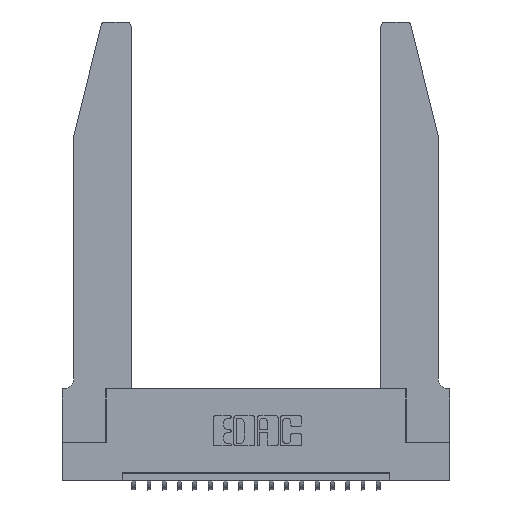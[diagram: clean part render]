
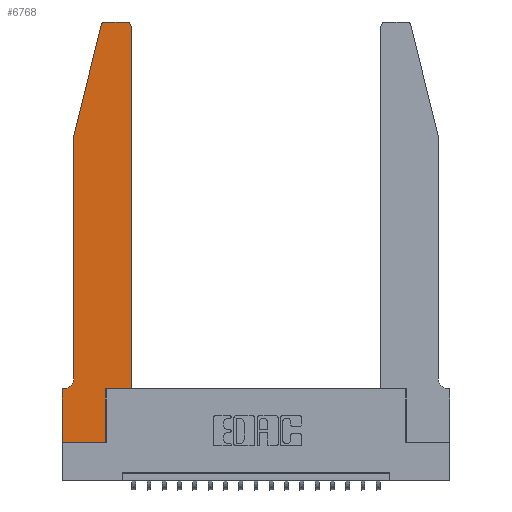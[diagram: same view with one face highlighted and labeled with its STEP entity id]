
A CAD part, top view. The second image highlights one B-rep face of the part: STEP entity #6768.
In plain terms, the highlighted planar face has unit normal (0, 0, 1).
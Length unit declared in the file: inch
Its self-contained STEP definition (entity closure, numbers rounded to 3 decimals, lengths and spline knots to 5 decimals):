
#66 = EDGE_CURVE ( 'NONE', #9543, #18279, #16035, .T. ) ;
#221 = VERTEX_POINT ( 'NONE', #3979 ) ;
#252 = DIRECTION ( 'NONE',  ( 0., -1., 0. ) ) ;
#942 = VERTEX_POINT ( 'NONE', #6035 ) ;
#1157 = CARTESIAN_POINT ( 'NONE',  ( 0.2865, 0., 0.37 ) ) ;
#1265 = EDGE_CURVE ( 'NONE', #18279, #14429, #11184, .T. ) ;
#2104 = ORIENTED_EDGE ( 'NONE', *, *, #1265, .T. ) ;
#2162 = LINE ( 'NONE', #9368, #5380 ) ;
#2373 = LINE ( 'NONE', #16168, #3080 ) ;
#2887 = CARTESIAN_POINT ( 'NONE',  ( 0., 0., 0.37 ) ) ;
#2983 = PLANE ( 'NONE',  #10038 ) ;
#3080 = VECTOR ( 'NONE', #16244, 39.37008 ) ;
#3248 = VERTEX_POINT ( 'NONE', #12413 ) ;
#3618 = CARTESIAN_POINT ( 'NONE',  ( 0.25487, 2.72718, 0.37 ) ) ;
#3940 = LINE ( 'NONE', #19467, #20176 ) ;
#3979 = CARTESIAN_POINT ( 'NONE',  ( 0., 0.35, 0.37 ) ) ;
#4299 = VECTOR ( 'NONE', #18456, 39.37008 ) ;
#4621 = EDGE_CURVE ( 'NONE', #221, #20211, #2162, .T. ) ;
#4654 = DIRECTION ( 'NONE',  ( 1., 0., 0. ) ) ;
#4764 = CARTESIAN_POINT ( 'NONE',  ( 0.0755, 0.42, 0.37 ) ) ;
#4888 = DIRECTION ( 'NONE',  ( -1., 0., 0. ) ) ;
#5045 = VECTOR ( 'NONE', #11213, 39.37008 ) ;
#5380 = VECTOR ( 'NONE', #20768, 39.37008 ) ;
#5398 = ORIENTED_EDGE ( 'NONE', *, *, #6050, .T. ) ;
#5723 = CARTESIAN_POINT ( 'NONE',  ( 0.0755, 2., 0.37 ) ) ;
#6035 = CARTESIAN_POINT ( 'NONE',  ( 0.4505, 0.35, 0.37 ) ) ;
#6050 = EDGE_CURVE ( 'NONE', #15713, #9543, #6128, .T. ) ;
#6083 = ORIENTED_EDGE ( 'NONE', *, *, #11339, .T. ) ;
#6128 = CIRCLE ( 'NONE', #12092, 0.03 ) ;
#6202 = DIRECTION ( 'NONE',  ( 0., 0., 1. ) ) ;
#6313 = CARTESIAN_POINT ( 'NONE',  ( 0.0755, 2., 0.37 ) ) ;
#6392 = ORIENTED_EDGE ( 'NONE', *, *, #66, .T. ) ;
#6768 = ADVANCED_FACE ( 'NONE', ( #17040 ), #2983, .T. ) ;
#6833 = VECTOR ( 'NONE', #17334, 39.37008 ) ;
#7091 = DIRECTION ( 'NONE',  ( 1., 0., 0. ) ) ;
#7896 = CARTESIAN_POINT ( 'NONE',  ( 0.4505, 0.35, 0.37 ) ) ;
#8015 = CARTESIAN_POINT ( 'NONE',  ( 0.2605, 2.75, 0.37 ) ) ;
#8116 = DIRECTION ( 'NONE',  ( 0., 0., 1. ) ) ;
#8284 = AXIS2_PLACEMENT_3D ( 'NONE', #12264, #16840, #7091 ) ;
#8472 = ORIENTED_EDGE ( 'NONE', *, *, #11374, .T. ) ;
#8602 = LINE ( 'NONE', #10929, #12241 ) ;
#8784 = ORIENTED_EDGE ( 'NONE', *, *, #14375, .T. ) ;
#9368 = CARTESIAN_POINT ( 'NONE',  ( 0., 0., 0.37 ) ) ;
#9543 = VERTEX_POINT ( 'NONE', #12449 ) ;
#9639 = DIRECTION ( 'NONE',  ( 1., 0., 0. ) ) ;
#9896 = VECTOR ( 'NONE', #18362, 39.37008 ) ;
#10038 = AXIS2_PLACEMENT_3D ( 'NONE', #16009, #6202, #9639 ) ;
#10655 = VERTEX_POINT ( 'NONE', #6313 ) ;
#10929 = CARTESIAN_POINT ( 'NONE',  ( 0.0755, 0.35, 0.37 ) ) ;
#11184 = CIRCLE ( 'NONE', #8284, 0.03 ) ;
#11213 = DIRECTION ( 'NONE',  ( 1., 0., 0. ) ) ;
#11339 = EDGE_CURVE ( 'NONE', #14429, #10655, #15521, .T. ) ;
#11374 = EDGE_CURVE ( 'NONE', #3248, #221, #8602, .T. ) ;
#11464 = CARTESIAN_POINT ( 'NONE',  ( 0.0055, 0.42, 0.37 ) ) ;
#12092 = AXIS2_PLACEMENT_3D ( 'NONE', #14551, #8116, #4654 ) ;
#12241 = VECTOR ( 'NONE', #18015, 39.37008 ) ;
#12264 = CARTESIAN_POINT ( 'NONE',  ( 0.284, 2.72, 0.37 ) ) ;
#12413 = CARTESIAN_POINT ( 'NONE',  ( 0.0055, 0.35, 0.37 ) ) ;
#12449 = CARTESIAN_POINT ( 'NONE',  ( 0.4205, 2.75, 0.37 ) ) ;
#12724 = VERTEX_POINT ( 'NONE', #1157 ) ;
#12768 = CARTESIAN_POINT ( 'NONE',  ( 0.284, 2.75, 0.37 ) ) ;
#13280 = ORIENTED_EDGE ( 'NONE', *, *, #13927, .T. ) ;
#13927 = EDGE_CURVE ( 'NONE', #18352, #3248, #14914, .T. ) ;
#13968 = ORIENTED_EDGE ( 'NONE', *, *, #14284, .T. ) ;
#14023 = ORIENTED_EDGE ( 'NONE', *, *, #4621, .T. ) ;
#14284 = EDGE_CURVE ( 'NONE', #20211, #12724, #2373, .T. ) ;
#14375 = EDGE_CURVE ( 'NONE', #10655, #18352, #3940, .T. ) ;
#14429 = VERTEX_POINT ( 'NONE', #3618 ) ;
#14551 = CARTESIAN_POINT ( 'NONE',  ( 0.4205, 2.72, 0.37 ) ) ;
#14659 = DIRECTION ( 'NONE',  ( 0., 0., -1. ) ) ;
#14764 = CARTESIAN_POINT ( 'NONE',  ( 0.4505, 2.72, 0.37 ) ) ;
#14914 = CIRCLE ( 'NONE', #15597, 0.07 ) ;
#15475 = EDGE_CURVE ( 'NONE', #942, #15713, #15994, .T. ) ;
#15521 = LINE ( 'NONE', #5723, #6833 ) ;
#15597 = AXIS2_PLACEMENT_3D ( 'NONE', #11464, #14659, #4888 ) ;
#15713 = VERTEX_POINT ( 'NONE', #14764 ) ;
#15779 = LINE ( 'NONE', #15984, #5045 ) ;
#15984 = CARTESIAN_POINT ( 'NONE',  ( 0.4505, 0.35, 0.37 ) ) ;
#15994 = LINE ( 'NONE', #7896, #18723 ) ;
#16009 = CARTESIAN_POINT ( 'NONE',  ( 0., 0.35, 0.37 ) ) ;
#16035 = LINE ( 'NONE', #8015, #9896 ) ;
#16168 = CARTESIAN_POINT ( 'NONE',  ( 0., 0., 0.37 ) ) ;
#16244 = DIRECTION ( 'NONE',  ( 1., 0., 0. ) ) ;
#16489 = EDGE_LOOP ( 'NONE', ( #6392, #2104, #6083, #8784, #13280, #8472, #14023, #13968, #16746, #17531, #17241, #5398 ) ) ;
#16746 = ORIENTED_EDGE ( 'NONE', *, *, #20513, .T. ) ;
#16840 = DIRECTION ( 'NONE',  ( 0., 0., 1. ) ) ;
#16852 = CARTESIAN_POINT ( 'NONE',  ( 0.2865, 0.35, 0.37 ) ) ;
#17040 = FACE_OUTER_BOUND ( 'NONE', #16489, .T. ) ;
#17241 = ORIENTED_EDGE ( 'NONE', *, *, #15475, .T. ) ;
#17334 = DIRECTION ( 'NONE',  ( -0.239, -0.971, 0. ) ) ;
#17531 = ORIENTED_EDGE ( 'NONE', *, *, #20244, .T. ) ;
#17638 = DIRECTION ( 'NONE',  ( 0., 1., 0. ) ) ;
#17998 = LINE ( 'NONE', #16852, #4299 ) ;
#18015 = DIRECTION ( 'NONE',  ( -1., 0., 0. ) ) ;
#18249 = VERTEX_POINT ( 'NONE', #20653 ) ;
#18279 = VERTEX_POINT ( 'NONE', #12768 ) ;
#18352 = VERTEX_POINT ( 'NONE', #4764 ) ;
#18362 = DIRECTION ( 'NONE',  ( -1., 0., 0. ) ) ;
#18456 = DIRECTION ( 'NONE',  ( 0., 1., 0. ) ) ;
#18723 = VECTOR ( 'NONE', #17638, 39.37008 ) ;
#19467 = CARTESIAN_POINT ( 'NONE',  ( 0.0755, 2., 0.37 ) ) ;
#20176 = VECTOR ( 'NONE', #252, 39.37008 ) ;
#20211 = VERTEX_POINT ( 'NONE', #2887 ) ;
#20244 = EDGE_CURVE ( 'NONE', #18249, #942, #15779, .T. ) ;
#20513 = EDGE_CURVE ( 'NONE', #12724, #18249, #17998, .T. ) ;
#20653 = CARTESIAN_POINT ( 'NONE',  ( 0.2865, 0.35, 0.37 ) ) ;
#20768 = DIRECTION ( 'NONE',  ( 0., -1., 0. ) ) ;
